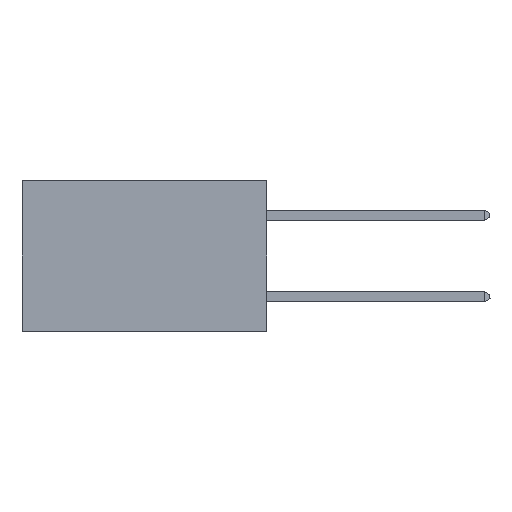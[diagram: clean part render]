
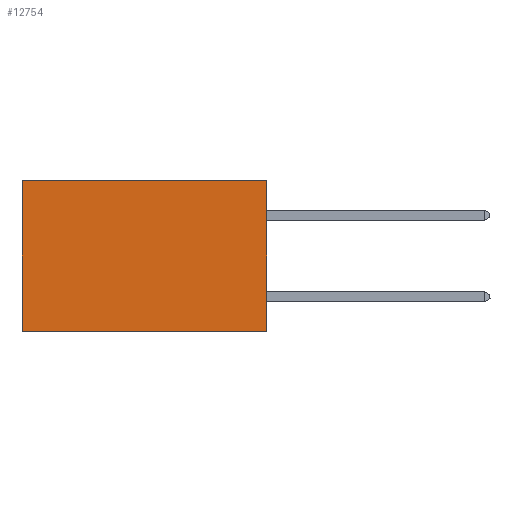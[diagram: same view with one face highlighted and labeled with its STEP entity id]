
A CAD part, left-side view. The second image highlights one B-rep face of the part: STEP entity #12754.
In plain terms, the highlighted planar face has unit normal (-1, 0, 0).
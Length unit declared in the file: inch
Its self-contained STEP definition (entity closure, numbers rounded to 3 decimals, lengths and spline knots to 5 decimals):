
#405 = CARTESIAN_POINT ( 'NONE',  ( 0.2875, 0.6, -0.37 ) ) ;
#656 = CARTESIAN_POINT ( 'NONE',  ( 0.2875, 0.6, 0. ) ) ;
#1238 = CARTESIAN_POINT ( 'NONE',  ( 0.2875, 0., -0.37 ) ) ;
#1785 = FACE_OUTER_BOUND ( 'NONE', #9192, .T. ) ;
#2817 = EDGE_CURVE ( 'NONE', #6121, #30195, #13320, .T. ) ;
#2880 = VECTOR ( 'NONE', #8371, 39.37008 ) ;
#3408 = AXIS2_PLACEMENT_3D ( 'NONE', #4812, #29988, #9624 ) ;
#3622 = EDGE_CURVE ( 'NONE', #6121, #4890, #9382, .T. ) ;
#4421 = VECTOR ( 'NONE', #13662, 39.37008 ) ;
#4462 = ORIENTED_EDGE ( 'NONE', *, *, #3622, .F. ) ;
#4812 = CARTESIAN_POINT ( 'NONE',  ( 0.2875, 0., 0. ) ) ;
#4890 = VERTEX_POINT ( 'NONE', #18219 ) ;
#5189 = CARTESIAN_POINT ( 'NONE',  ( 0.2875, 0., 0. ) ) ;
#5522 = ORIENTED_EDGE ( 'NONE', *, *, #21262, .F. ) ;
#5865 = CARTESIAN_POINT ( 'NONE',  ( 0.2875, 0.6, 0. ) ) ;
#6121 = VERTEX_POINT ( 'NONE', #16638 ) ;
#8371 = DIRECTION ( 'NONE',  ( 0., 0., -1. ) ) ;
#9111 = CARTESIAN_POINT ( 'NONE',  ( 0.2875, 0., 0. ) ) ;
#9192 = EDGE_LOOP ( 'NONE', ( #11203, #5522, #4462, #16192 ) ) ;
#9225 = DIRECTION ( 'NONE',  ( 0., 1., 0. ) ) ;
#9382 = LINE ( 'NONE', #5189, #20587 ) ;
#9438 = VECTOR ( 'NONE', #9225, 39.37008 ) ;
#9624 = DIRECTION ( 'NONE',  ( 0., 0., -1. ) ) ;
#11203 = ORIENTED_EDGE ( 'NONE', *, *, #25649, .T. ) ;
#12754 = ADVANCED_FACE ( 'NONE', ( #1785 ), #28072, .F. ) ;
#13320 = LINE ( 'NONE', #9111, #9438 ) ;
#13662 = DIRECTION ( 'NONE',  ( 0., 1., 0. ) ) ;
#13754 = LINE ( 'NONE', #1238, #4421 ) ;
#16192 = ORIENTED_EDGE ( 'NONE', *, *, #2817, .T. ) ;
#16638 = CARTESIAN_POINT ( 'NONE',  ( 0.2875, 0., 0. ) ) ;
#18219 = CARTESIAN_POINT ( 'NONE',  ( 0.2875, 0., -0.37 ) ) ;
#20587 = VECTOR ( 'NONE', #22536, 39.37008 ) ;
#21262 = EDGE_CURVE ( 'NONE', #4890, #23522, #13754, .T. ) ;
#22536 = DIRECTION ( 'NONE',  ( 0., 0., -1. ) ) ;
#23522 = VERTEX_POINT ( 'NONE', #405 ) ;
#23845 = LINE ( 'NONE', #5865, #2880 ) ;
#25649 = EDGE_CURVE ( 'NONE', #30195, #23522, #23845, .T. ) ;
#28072 = PLANE ( 'NONE',  #3408 ) ;
#29988 = DIRECTION ( 'NONE',  ( 1., 0., 0. ) ) ;
#30195 = VERTEX_POINT ( 'NONE', #656 ) ;
